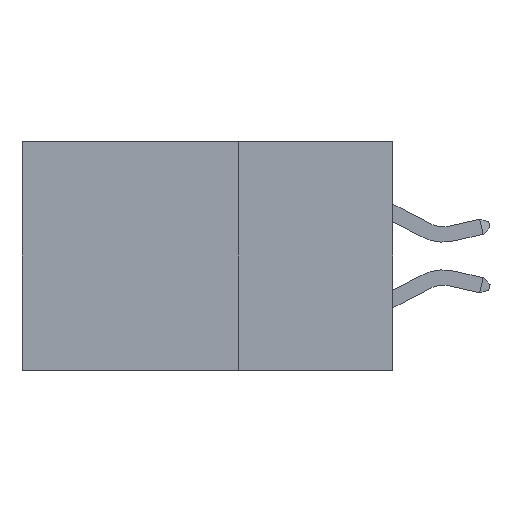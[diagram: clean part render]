
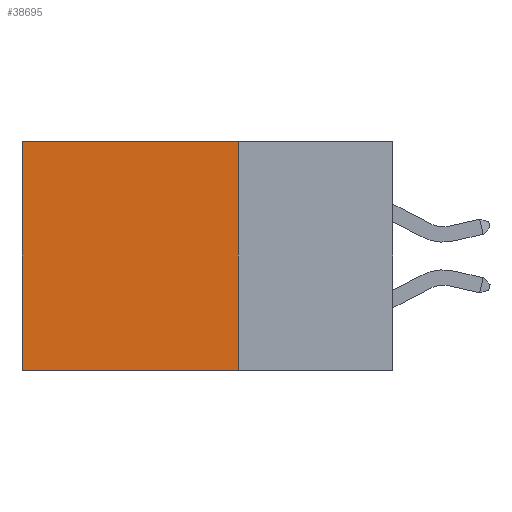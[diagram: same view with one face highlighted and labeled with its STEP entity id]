
A CAD part, left-side view. The second image highlights one B-rep face of the part: STEP entity #38695.
In plain terms, the highlighted planar face has unit normal (-1, 0, 0).
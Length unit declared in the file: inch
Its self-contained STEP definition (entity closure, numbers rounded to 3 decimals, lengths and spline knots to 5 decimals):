
#98 = CARTESIAN_POINT ( 'NONE',  ( 0.2875, 0.6, -0.37 ) ) ;
#969 = DIRECTION ( 'NONE',  ( 1., 0., 0. ) ) ;
#1665 = VECTOR ( 'NONE', #2509, 39.37008 ) ;
#2509 = DIRECTION ( 'NONE',  ( 0., 1., 0. ) ) ;
#2691 = CARTESIAN_POINT ( 'NONE',  ( 0.2875, 0.6, 0. ) ) ;
#3941 = CARTESIAN_POINT ( 'NONE',  ( 0.2875, 0.25, 0. ) ) ;
#5259 = EDGE_LOOP ( 'NONE', ( #29246, #17060, #36431, #23586 ) ) ;
#5979 = LINE ( 'NONE', #2691, #33301 ) ;
#6135 = VERTEX_POINT ( 'NONE', #3941 ) ;
#6685 = EDGE_CURVE ( 'NONE', #32675, #17753, #5979, .T. ) ;
#6960 = FACE_OUTER_BOUND ( 'NONE', #5259, .T. ) ;
#11822 = EDGE_CURVE ( 'NONE', #6135, #23670, #29014, .T. ) ;
#11933 = EDGE_CURVE ( 'NONE', #23670, #17753, #15597, .T. ) ;
#15597 = LINE ( 'NONE', #29978, #1665 ) ;
#16641 = VECTOR ( 'NONE', #23739, 39.37008 ) ;
#17060 = ORIENTED_EDGE ( 'NONE', *, *, #11933, .F. ) ;
#17699 = EDGE_CURVE ( 'NONE', #6135, #32675, #32419, .T. ) ;
#17753 = VERTEX_POINT ( 'NONE', #98 ) ;
#19356 = CARTESIAN_POINT ( 'NONE',  ( 0.2875, 0.25, 0. ) ) ;
#20757 = CARTESIAN_POINT ( 'NONE',  ( 0.2875, 0.25, 0. ) ) ;
#23268 = VECTOR ( 'NONE', #30342, 39.37008 ) ;
#23586 = ORIENTED_EDGE ( 'NONE', *, *, #17699, .T. ) ;
#23670 = VERTEX_POINT ( 'NONE', #24624 ) ;
#23739 = DIRECTION ( 'NONE',  ( 0., 1., 0. ) ) ;
#24130 = CARTESIAN_POINT ( 'NONE',  ( 0.2875, 0.25, 0. ) ) ;
#24462 = CARTESIAN_POINT ( 'NONE',  ( 0.2875, 0.6, 0. ) ) ;
#24624 = CARTESIAN_POINT ( 'NONE',  ( 0.2875, 0.25, -0.37 ) ) ;
#28434 = PLANE ( 'NONE',  #34873 ) ;
#28579 = DIRECTION ( 'NONE',  ( 0., 0., -1. ) ) ;
#29014 = LINE ( 'NONE', #20757, #23268 ) ;
#29246 = ORIENTED_EDGE ( 'NONE', *, *, #6685, .T. ) ;
#29978 = CARTESIAN_POINT ( 'NONE',  ( 0.2875, 0.25, -0.37 ) ) ;
#30342 = DIRECTION ( 'NONE',  ( 0., 0., -1. ) ) ;
#32419 = LINE ( 'NONE', #24130, #16641 ) ;
#32675 = VERTEX_POINT ( 'NONE', #24462 ) ;
#33301 = VECTOR ( 'NONE', #33564, 39.37008 ) ;
#33564 = DIRECTION ( 'NONE',  ( 0., 0., -1. ) ) ;
#34873 = AXIS2_PLACEMENT_3D ( 'NONE', #19356, #969, #28579 ) ;
#36431 = ORIENTED_EDGE ( 'NONE', *, *, #11822, .F. ) ;
#38695 = ADVANCED_FACE ( 'NONE', ( #6960 ), #28434, .F. ) ;
